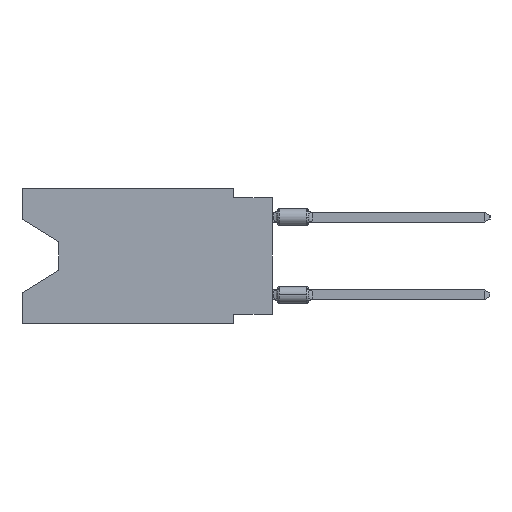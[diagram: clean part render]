
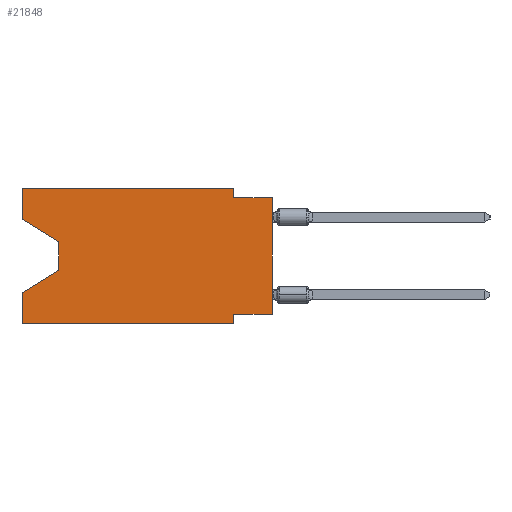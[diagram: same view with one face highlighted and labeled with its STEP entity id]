
A CAD part, left-side view. The second image highlights one B-rep face of the part: STEP entity #21848.
In plain terms, the highlighted planar face has unit normal (-1, 0, 0).
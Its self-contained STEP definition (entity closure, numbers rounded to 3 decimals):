
#747 = EDGE_CURVE ( 'NONE', #18358, #41854, #5771, .T. ) ;
#1695 = VERTEX_POINT ( 'NONE', #55700 ) ;
#2905 = VECTOR ( 'NONE', #11877, 1000. ) ;
#4838 = VECTOR ( 'NONE', #17537, 1000. ) ;
#5176 = CARTESIAN_POINT ( 'NONE',  ( 0., 16.383, 0. ) ) ;
#5771 = LINE ( 'NONE', #26080, #24216 ) ;
#5830 = CARTESIAN_POINT ( 'NONE',  ( 0., 2.54, -8.255 ) ) ;
#6340 = CARTESIAN_POINT ( 'NONE',  ( 0., 16.383, 0. ) ) ;
#6688 = EDGE_CURVE ( 'NONE', #1695, #14906, #31817, .T. ) ;
#6847 = CARTESIAN_POINT ( 'NONE',  ( 0., 16.383, -2.038 ) ) ;
#7863 = LINE ( 'NONE', #13208, #4838 ) ;
#8168 = LINE ( 'NONE', #58106, #2905 ) ;
#8919 = EDGE_CURVE ( 'NONE', #15280, #20804, #39592, .T. ) ;
#9136 = ORIENTED_EDGE ( 'NONE', *, *, #18092, .F. ) ;
#9871 = DIRECTION ( 'NONE',  ( 0., -1., 0. ) ) ;
#10796 = EDGE_CURVE ( 'NONE', #15280, #12580, #14871, .T. ) ;
#11194 = VECTOR ( 'NONE', #60716, 1000. ) ;
#11877 = DIRECTION ( 'NONE',  ( 0., 0.855, -0.519 ) ) ;
#12580 = VERTEX_POINT ( 'NONE', #38061 ) ;
#13208 = CARTESIAN_POINT ( 'NONE',  ( 0., 16.383, 0. ) ) ;
#14437 = VERTEX_POINT ( 'NONE', #23101 ) ;
#14714 = EDGE_CURVE ( 'NONE', #1695, #14437, #51929, .T. ) ;
#14871 = LINE ( 'NONE', #55446, #32692 ) ;
#14906 = VERTEX_POINT ( 'NONE', #44237 ) ;
#15280 = VERTEX_POINT ( 'NONE', #29185 ) ;
#15284 = VECTOR ( 'NONE', #27693, 1000. ) ;
#15950 = ORIENTED_EDGE ( 'NONE', *, *, #14714, .F. ) ;
#17537 = DIRECTION ( 'NONE',  ( 0., -1., 0. ) ) ;
#17593 = VECTOR ( 'NONE', #46773, 1000. ) ;
#17718 = LINE ( 'NONE', #42990, #15284 ) ;
#18092 = EDGE_CURVE ( 'NONE', #23760, #22847, #17718, .T. ) ;
#18358 = VERTEX_POINT ( 'NONE', #44974 ) ;
#19528 = DIRECTION ( 'NONE',  ( 1., 0., 0. ) ) ;
#20804 = VERTEX_POINT ( 'NONE', #22435 ) ;
#21306 = VERTEX_POINT ( 'NONE', #35229 ) ;
#21460 = ORIENTED_EDGE ( 'NONE', *, *, #62640, .T. ) ;
#21804 = AXIS2_PLACEMENT_3D ( 'NONE', #5176, #19528, #60098 ) ;
#21848 = ADVANCED_FACE ( 'NONE', ( #50760 ), #34504, .F. ) ;
#22435 = CARTESIAN_POINT ( 'NONE',  ( 0., 16.383, -6.852 ) ) ;
#22480 = VECTOR ( 'NONE', #42805, 1000. ) ;
#22593 = EDGE_CURVE ( 'NONE', #14437, #18358, #7863, .T. ) ;
#22847 = VERTEX_POINT ( 'NONE', #5830 ) ;
#23101 = CARTESIAN_POINT ( 'NONE',  ( 0., 16.383, 0. ) ) ;
#23366 = ORIENTED_EDGE ( 'NONE', *, *, #6688, .T. ) ;
#23760 = VERTEX_POINT ( 'NONE', #43138 ) ;
#24187 = LINE ( 'NONE', #48477, #34457 ) ;
#24216 = VECTOR ( 'NONE', #46350, 1000. ) ;
#26080 = CARTESIAN_POINT ( 'NONE',  ( 0., 2.54, 0. ) ) ;
#26647 = DIRECTION ( 'NONE',  ( 0., 0., 1. ) ) ;
#27693 = DIRECTION ( 'NONE',  ( 0., 1., 0. ) ) ;
#29117 = VERTEX_POINT ( 'NONE', #46997 ) ;
#29153 = EDGE_LOOP ( 'NONE', ( #23366, #21460, #54168, #47106, #60788, #47188, #9136, #57151, #51458, #48481, #30677, #15950 ) ) ;
#29185 = CARTESIAN_POINT ( 'NONE',  ( 0., 16.383, -8.89 ) ) ;
#30677 = ORIENTED_EDGE ( 'NONE', *, *, #22593, .F. ) ;
#30790 = CARTESIAN_POINT ( 'NONE',  ( 0., 0., 0. ) ) ;
#31374 = EDGE_CURVE ( 'NONE', #41854, #21306, #37482, .T. ) ;
#31817 = LINE ( 'NONE', #6847, #17593 ) ;
#32139 = VECTOR ( 'NONE', #26647, 1000. ) ;
#32676 = EDGE_CURVE ( 'NONE', #23760, #21306, #36100, .T. ) ;
#32692 = VECTOR ( 'NONE', #9871, 1000. ) ;
#34457 = VECTOR ( 'NONE', #58470, 1000. ) ;
#34504 = PLANE ( 'NONE',  #21804 ) ;
#35229 = CARTESIAN_POINT ( 'NONE',  ( 0., 0., -0.635 ) ) ;
#35262 = CARTESIAN_POINT ( 'NONE',  ( 0., 16.383, 0. ) ) ;
#35746 = EDGE_CURVE ( 'NONE', #29117, #20804, #8168, .T. ) ;
#36100 = LINE ( 'NONE', #30790, #11194 ) ;
#37482 = LINE ( 'NONE', #58111, #22480 ) ;
#38061 = CARTESIAN_POINT ( 'NONE',  ( 0., 2.54, -8.89 ) ) ;
#39592 = LINE ( 'NONE', #35262, #42177 ) ;
#41854 = VERTEX_POINT ( 'NONE', #42940 ) ;
#42177 = VECTOR ( 'NONE', #54577, 1000. ) ;
#42805 = DIRECTION ( 'NONE',  ( 0., -1., 0. ) ) ;
#42940 = CARTESIAN_POINT ( 'NONE',  ( 0., 2.54, -0.635 ) ) ;
#42990 = CARTESIAN_POINT ( 'NONE',  ( 0., 0., -8.255 ) ) ;
#43138 = CARTESIAN_POINT ( 'NONE',  ( 0., 0., -8.255 ) ) ;
#44237 = CARTESIAN_POINT ( 'NONE',  ( 0., 13.97, -3.505 ) ) ;
#44974 = CARTESIAN_POINT ( 'NONE',  ( 0., 2.54, 0. ) ) ;
#46350 = DIRECTION ( 'NONE',  ( 0., 0., -1. ) ) ;
#46773 = DIRECTION ( 'NONE',  ( 0., -0.855, -0.519 ) ) ;
#46997 = CARTESIAN_POINT ( 'NONE',  ( 0., 13.97, -5.385 ) ) ;
#47106 = ORIENTED_EDGE ( 'NONE', *, *, #8919, .F. ) ;
#47188 = ORIENTED_EDGE ( 'NONE', *, *, #50513, .F. ) ;
#48477 = CARTESIAN_POINT ( 'NONE',  ( 0., 2.54, -8.89 ) ) ;
#48481 = ORIENTED_EDGE ( 'NONE', *, *, #747, .F. ) ;
#50513 = EDGE_CURVE ( 'NONE', #22847, #12580, #24187, .T. ) ;
#50760 = FACE_OUTER_BOUND ( 'NONE', #29153, .T. ) ;
#51458 = ORIENTED_EDGE ( 'NONE', *, *, #31374, .F. ) ;
#51929 = LINE ( 'NONE', #6340, #32139 ) ;
#54168 = ORIENTED_EDGE ( 'NONE', *, *, #35746, .T. ) ;
#54577 = DIRECTION ( 'NONE',  ( 0., 0., 1. ) ) ;
#55446 = CARTESIAN_POINT ( 'NONE',  ( 0., 16.383, -8.89 ) ) ;
#55700 = CARTESIAN_POINT ( 'NONE',  ( 0., 16.383, -2.038 ) ) ;
#56274 = DIRECTION ( 'NONE',  ( 0., 0., -1. ) ) ;
#57151 = ORIENTED_EDGE ( 'NONE', *, *, #32676, .T. ) ;
#57579 = CARTESIAN_POINT ( 'NONE',  ( 0., 13.97, -3.505 ) ) ;
#58106 = CARTESIAN_POINT ( 'NONE',  ( 0., 13.97, -5.385 ) ) ;
#58111 = CARTESIAN_POINT ( 'NONE',  ( 0., 0., -0.635 ) ) ;
#58470 = DIRECTION ( 'NONE',  ( 0., 0., -1. ) ) ;
#59485 = VECTOR ( 'NONE', #56274, 1000. ) ;
#60098 = DIRECTION ( 'NONE',  ( 0., 0., -1. ) ) ;
#60716 = DIRECTION ( 'NONE',  ( 0., 0., 1. ) ) ;
#60788 = ORIENTED_EDGE ( 'NONE', *, *, #10796, .T. ) ;
#62582 = LINE ( 'NONE', #57579, #59485 ) ;
#62640 = EDGE_CURVE ( 'NONE', #14906, #29117, #62582, .T. ) ;
